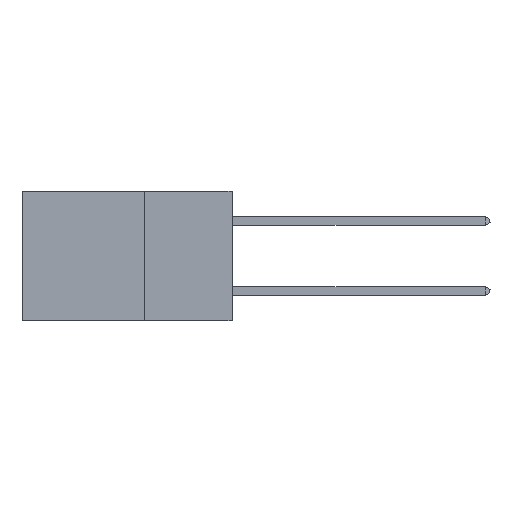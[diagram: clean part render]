
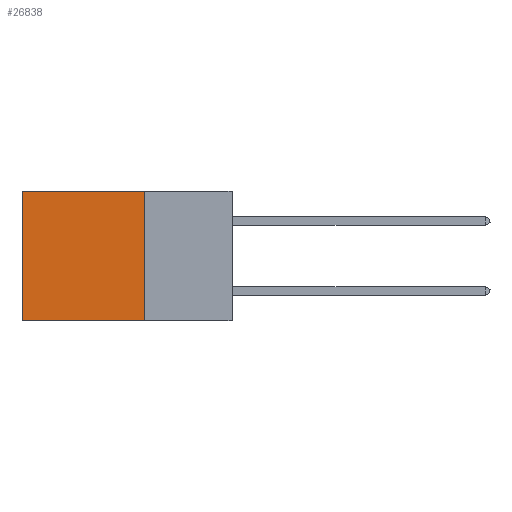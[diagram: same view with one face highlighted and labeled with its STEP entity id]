
A CAD part, left-side view. The second image highlights one B-rep face of the part: STEP entity #26838.
In plain terms, the highlighted planar face has unit normal (-1, 0, 0).
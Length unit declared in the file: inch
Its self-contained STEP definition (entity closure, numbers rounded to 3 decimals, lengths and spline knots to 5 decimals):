
#298 = DIRECTION ( 'NONE',  ( 0., 1., 0. ) ) ;
#546 = CARTESIAN_POINT ( 'NONE',  ( 0.2875, 0.25, 0. ) ) ;
#2691 = PLANE ( 'NONE',  #3818 ) ;
#2790 = DIRECTION ( 'NONE',  ( 0., 0., -1. ) ) ;
#3818 = AXIS2_PLACEMENT_3D ( 'NONE', #546, #15542, #2790 ) ;
#4699 = EDGE_CURVE ( 'NONE', #16403, #16356, #7614, .T. ) ;
#5812 = DIRECTION ( 'NONE',  ( 0., 0., -1. ) ) ;
#6812 = LINE ( 'NONE', #11939, #7513 ) ;
#6992 = EDGE_CURVE ( 'NONE', #14822, #9379, #7478, .T. ) ;
#7478 = LINE ( 'NONE', #8710, #8176 ) ;
#7513 = VECTOR ( 'NONE', #26596, 39.37008 ) ;
#7614 = LINE ( 'NONE', #14259, #12585 ) ;
#8176 = VECTOR ( 'NONE', #10851, 39.37008 ) ;
#8710 = CARTESIAN_POINT ( 'NONE',  ( 0.2875, 0.25, 0. ) ) ;
#8780 = ORIENTED_EDGE ( 'NONE', *, *, #17491, .T. ) ;
#9379 = VERTEX_POINT ( 'NONE', #20044 ) ;
#10494 = FACE_OUTER_BOUND ( 'NONE', #22247, .T. ) ;
#10851 = DIRECTION ( 'NONE',  ( 0., 0., -1. ) ) ;
#11939 = CARTESIAN_POINT ( 'NONE',  ( 0.2875, 0.25, -0.37 ) ) ;
#12585 = VECTOR ( 'NONE', #5812, 39.37008 ) ;
#14259 = CARTESIAN_POINT ( 'NONE',  ( 0.2875, 0.6, 0. ) ) ;
#14438 = ORIENTED_EDGE ( 'NONE', *, *, #16386, .F. ) ;
#14822 = VERTEX_POINT ( 'NONE', #17135 ) ;
#15281 = CARTESIAN_POINT ( 'NONE',  ( 0.2875, 0.25, 0. ) ) ;
#15542 = DIRECTION ( 'NONE',  ( 1., 0., 0. ) ) ;
#16356 = VERTEX_POINT ( 'NONE', #20199 ) ;
#16386 = EDGE_CURVE ( 'NONE', #9379, #16356, #6812, .T. ) ;
#16403 = VERTEX_POINT ( 'NONE', #24513 ) ;
#17135 = CARTESIAN_POINT ( 'NONE',  ( 0.2875, 0.25, 0. ) ) ;
#17491 = EDGE_CURVE ( 'NONE', #14822, #16403, #22633, .T. ) ;
#17507 = ORIENTED_EDGE ( 'NONE', *, *, #4699, .T. ) ;
#19273 = ORIENTED_EDGE ( 'NONE', *, *, #6992, .F. ) ;
#20044 = CARTESIAN_POINT ( 'NONE',  ( 0.2875, 0.25, -0.37 ) ) ;
#20199 = CARTESIAN_POINT ( 'NONE',  ( 0.2875, 0.6, -0.37 ) ) ;
#21280 = VECTOR ( 'NONE', #298, 39.37008 ) ;
#22247 = EDGE_LOOP ( 'NONE', ( #17507, #14438, #19273, #8780 ) ) ;
#22633 = LINE ( 'NONE', #15281, #21280 ) ;
#24513 = CARTESIAN_POINT ( 'NONE',  ( 0.2875, 0.6, 0. ) ) ;
#26596 = DIRECTION ( 'NONE',  ( 0., 1., 0. ) ) ;
#26838 = ADVANCED_FACE ( 'NONE', ( #10494 ), #2691, .F. ) ;
